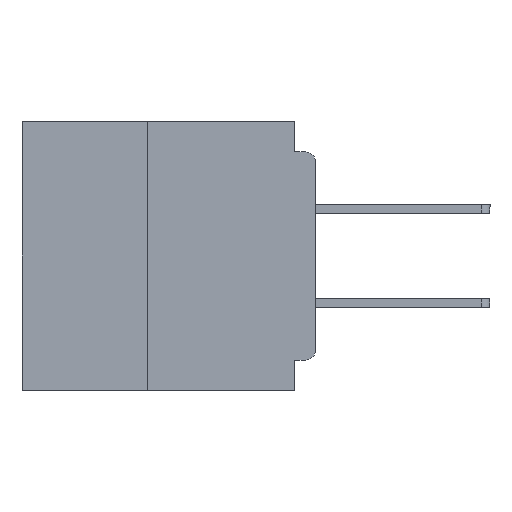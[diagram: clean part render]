
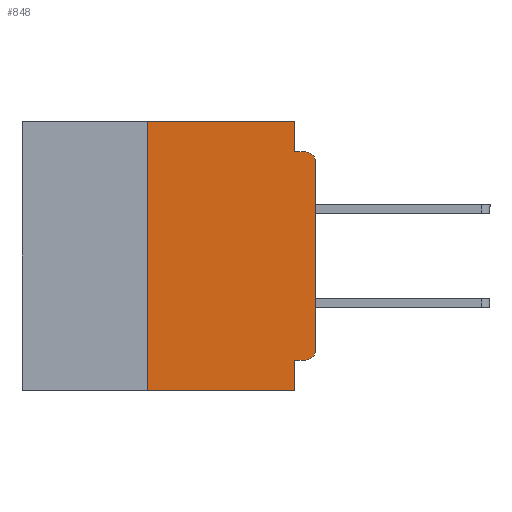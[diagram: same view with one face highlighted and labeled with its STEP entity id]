
A CAD part, left-side view. The second image highlights one B-rep face of the part: STEP entity #848.
In plain terms, the highlighted planar face has unit normal (-1, 0, 0).
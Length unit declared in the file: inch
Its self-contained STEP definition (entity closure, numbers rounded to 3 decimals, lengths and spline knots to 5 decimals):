
#105 = CIRCLE ( 'NONE', #41516, 0.015 ) ;
#127 = CARTESIAN_POINT ( 'NONE',  ( 0., 0., -0.06 ) ) ;
#433 = VERTEX_POINT ( 'NONE', #15902 ) ;
#518 = DIRECTION ( 'NONE',  ( 0., 0., 1. ) ) ;
#848 = ADVANCED_FACE ( 'NONE', ( #43755 ), #47490, .F. ) ;
#1095 = CARTESIAN_POINT ( 'NONE',  ( 0., 0.015, -0.045 ) ) ;
#2011 = CARTESIAN_POINT ( 'NONE',  ( 0., 0.031, -0.4 ) ) ;
#2278 = EDGE_CURVE ( 'NONE', #13363, #433, #6837, .T. ) ;
#2956 = VERTEX_POINT ( 'NONE', #127 ) ;
#3980 = ORIENTED_EDGE ( 'NONE', *, *, #23060, .F. ) ;
#4319 = EDGE_CURVE ( 'NONE', #46608, #22799, #13374, .T. ) ;
#4724 = DIRECTION ( 'NONE',  ( 0., -1., 0. ) ) ;
#5073 = DIRECTION ( 'NONE',  ( 0., -1., 0. ) ) ;
#5468 = CARTESIAN_POINT ( 'NONE',  ( 0., 0.437, -0.4 ) ) ;
#5474 = CARTESIAN_POINT ( 'NONE',  ( 0., 0., -0.355 ) ) ;
#6590 = VECTOR ( 'NONE', #18258, 39.37008 ) ;
#6837 = LINE ( 'NONE', #5468, #35178 ) ;
#7018 = CARTESIAN_POINT ( 'NONE',  ( 0., 0.031, -0.045 ) ) ;
#10385 = DIRECTION ( 'NONE',  ( 0., 0., 1. ) ) ;
#12143 = VECTOR ( 'NONE', #4724, 39.37008 ) ;
#13363 = VERTEX_POINT ( 'NONE', #25791 ) ;
#13374 = LINE ( 'NONE', #35611, #12143 ) ;
#13389 = DIRECTION ( 'NONE',  ( -1., 0., 0. ) ) ;
#13412 = CIRCLE ( 'NONE', #46250, 0.015 ) ;
#13458 = ORIENTED_EDGE ( 'NONE', *, *, #32583, .F. ) ;
#15610 = VECTOR ( 'NONE', #29055, 39.37008 ) ;
#15720 = EDGE_CURVE ( 'NONE', #2956, #22799, #105, .T. ) ;
#15902 = CARTESIAN_POINT ( 'NONE',  ( 0., 0.031, -0.4 ) ) ;
#17381 = DIRECTION ( 'NONE',  ( -1., 0., 0. ) ) ;
#18258 = DIRECTION ( 'NONE',  ( 0., 0., -1. ) ) ;
#18470 = VERTEX_POINT ( 'NONE', #22723 ) ;
#19188 = ORIENTED_EDGE ( 'NONE', *, *, #49613, .F. ) ;
#19880 = CARTESIAN_POINT ( 'NONE',  ( 0., 0., 0. ) ) ;
#20493 = EDGE_CURVE ( 'NONE', #13363, #18470, #25778, .T. ) ;
#20672 = ORIENTED_EDGE ( 'NONE', *, *, #2278, .T. ) ;
#22549 = EDGE_CURVE ( 'NONE', #44951, #2956, #39784, .T. ) ;
#22723 = CARTESIAN_POINT ( 'NONE',  ( 0., 0.25, 0. ) ) ;
#22799 = VERTEX_POINT ( 'NONE', #1095 ) ;
#22952 = VERTEX_POINT ( 'NONE', #36694 ) ;
#23060 = EDGE_CURVE ( 'NONE', #35509, #46608, #36138, .T. ) ;
#23531 = VECTOR ( 'NONE', #45908, 39.37008 ) ;
#23963 = VECTOR ( 'NONE', #40203, 39.37008 ) ;
#24687 = LINE ( 'NONE', #2011, #15610 ) ;
#25778 = LINE ( 'NONE', #48655, #26946 ) ;
#25791 = CARTESIAN_POINT ( 'NONE',  ( 0., 0.25, -0.4 ) ) ;
#26946 = VECTOR ( 'NONE', #10385, 39.37008 ) ;
#27961 = CARTESIAN_POINT ( 'NONE',  ( 0., 0.031, 0. ) ) ;
#28643 = EDGE_CURVE ( 'NONE', #33778, #22952, #35323, .T. ) ;
#29055 = DIRECTION ( 'NONE',  ( 0., 0., -1. ) ) ;
#29630 = VECTOR ( 'NONE', #518, 39.37008 ) ;
#30347 = ORIENTED_EDGE ( 'NONE', *, *, #4319, .F. ) ;
#30556 = CARTESIAN_POINT ( 'NONE',  ( 0., 0.437, 0. ) ) ;
#31524 = ORIENTED_EDGE ( 'NONE', *, *, #22549, .T. ) ;
#31828 = EDGE_LOOP ( 'NONE', ( #31524, #41667, #30347, #3980, #13458, #46702, #20672, #19188, #39925, #49284 ) ) ;
#32583 = EDGE_CURVE ( 'NONE', #18470, #35509, #45087, .T. ) ;
#33778 = VERTEX_POINT ( 'NONE', #42313 ) ;
#35178 = VECTOR ( 'NONE', #5073, 39.37008 ) ;
#35246 = CARTESIAN_POINT ( 'NONE',  ( 0., 0., -0.34 ) ) ;
#35323 = LINE ( 'NONE', #5474, #23963 ) ;
#35509 = VERTEX_POINT ( 'NONE', #27961 ) ;
#35611 = CARTESIAN_POINT ( 'NONE',  ( 0., 0., -0.045 ) ) ;
#36138 = LINE ( 'NONE', #41196, #6590 ) ;
#36447 = CARTESIAN_POINT ( 'NONE',  ( 0., 0.015, -0.34 ) ) ;
#36694 = CARTESIAN_POINT ( 'NONE',  ( 0., 0.031, -0.355 ) ) ;
#37596 = AXIS2_PLACEMENT_3D ( 'NONE', #47099, #46933, #46816 ) ;
#39784 = LINE ( 'NONE', #19880, #29630 ) ;
#39925 = ORIENTED_EDGE ( 'NONE', *, *, #28643, .F. ) ;
#40203 = DIRECTION ( 'NONE',  ( 0., 1., 0. ) ) ;
#40290 = DIRECTION ( 'NONE',  ( 0., 0., -1. ) ) ;
#40347 = CARTESIAN_POINT ( 'NONE',  ( 0., 0.015, -0.06 ) ) ;
#41196 = CARTESIAN_POINT ( 'NONE',  ( 0., 0.031, 0. ) ) ;
#41516 = AXIS2_PLACEMENT_3D ( 'NONE', #40347, #17381, #44176 ) ;
#41667 = ORIENTED_EDGE ( 'NONE', *, *, #15720, .T. ) ;
#42313 = CARTESIAN_POINT ( 'NONE',  ( 0., 0.015, -0.355 ) ) ;
#43755 = FACE_OUTER_BOUND ( 'NONE', #31828, .T. ) ;
#44176 = DIRECTION ( 'NONE',  ( 0., 0., -1. ) ) ;
#44951 = VERTEX_POINT ( 'NONE', #35246 ) ;
#45087 = LINE ( 'NONE', #30556, #23531 ) ;
#45908 = DIRECTION ( 'NONE',  ( 0., -1., 0. ) ) ;
#46250 = AXIS2_PLACEMENT_3D ( 'NONE', #36447, #13389, #40290 ) ;
#46608 = VERTEX_POINT ( 'NONE', #7018 ) ;
#46702 = ORIENTED_EDGE ( 'NONE', *, *, #20493, .F. ) ;
#46816 = DIRECTION ( 'NONE',  ( 0., 0., -1. ) ) ;
#46933 = DIRECTION ( 'NONE',  ( 1., 0., 0. ) ) ;
#47099 = CARTESIAN_POINT ( 'NONE',  ( 0., 0.437, 0. ) ) ;
#47490 = PLANE ( 'NONE',  #37596 ) ;
#47508 = EDGE_CURVE ( 'NONE', #33778, #44951, #13412, .T. ) ;
#48655 = CARTESIAN_POINT ( 'NONE',  ( 0., 0.25, -0.4 ) ) ;
#49284 = ORIENTED_EDGE ( 'NONE', *, *, #47508, .T. ) ;
#49613 = EDGE_CURVE ( 'NONE', #22952, #433, #24687, .T. ) ;
